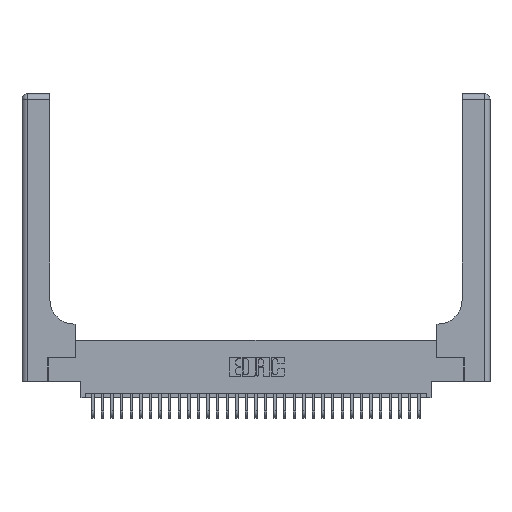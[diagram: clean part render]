
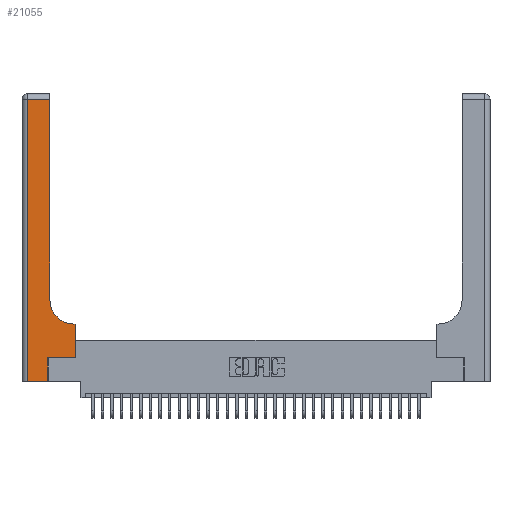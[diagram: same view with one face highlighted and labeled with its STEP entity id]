
A CAD part, top view. The second image highlights one B-rep face of the part: STEP entity #21055.
In plain terms, the highlighted planar face has unit normal (0, 0, 1).
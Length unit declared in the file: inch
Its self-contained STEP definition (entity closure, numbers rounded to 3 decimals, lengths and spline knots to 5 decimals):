
#862 = VECTOR ( 'NONE', #19435, 39.37008 ) ;
#910 = VECTOR ( 'NONE', #25590, 39.37008 ) ;
#3009 = CARTESIAN_POINT ( 'NONE',  ( 0.2915, 3., 0.37 ) ) ;
#3284 = VERTEX_POINT ( 'NONE', #5786 ) ;
#3422 = LINE ( 'NONE', #10126, #9938 ) ;
#4030 = VERTEX_POINT ( 'NONE', #9786 ) ;
#4068 = ORIENTED_EDGE ( 'NONE', *, *, #33892, .T. ) ;
#4175 = CARTESIAN_POINT ( 'NONE',  ( 0.5585, 0.25, 0.37 ) ) ;
#4227 = EDGE_CURVE ( 'NONE', #10998, #13736, #13913, .T. ) ;
#4533 = ORIENTED_EDGE ( 'NONE', *, *, #24375, .T. ) ;
#4627 = EDGE_CURVE ( 'NONE', #26095, #4030, #8307, .T. ) ;
#5786 = CARTESIAN_POINT ( 'NONE',  ( 0.269, 0., 0.37 ) ) ;
#6485 = CARTESIAN_POINT ( 'NONE',  ( 0.06, 3., 0.37 ) ) ;
#7587 = CARTESIAN_POINT ( 'NONE',  ( 0.2915, 0.85, 0.37 ) ) ;
#7722 = CARTESIAN_POINT ( 'NONE',  ( 0., 2.94, 0.37 ) ) ;
#8307 = LINE ( 'NONE', #6485, #910 ) ;
#9136 = CARTESIAN_POINT ( 'NONE',  ( 0.5415, 0.85, 0.37 ) ) ;
#9786 = CARTESIAN_POINT ( 'NONE',  ( 0.06, 0., 0.37 ) ) ;
#9938 = VECTOR ( 'NONE', #26439, 39.37008 ) ;
#10126 = CARTESIAN_POINT ( 'NONE',  ( 0., 0., 0.37 ) ) ;
#10458 = LINE ( 'NONE', #11432, #16880 ) ;
#10578 = ORIENTED_EDGE ( 'NONE', *, *, #33501, .T. ) ;
#10711 = EDGE_LOOP ( 'NONE', ( #10578, #4533, #21641, #4068, #14881, #26355, #33991, #20847, #14951 ) ) ;
#10998 = VERTEX_POINT ( 'NONE', #25466 ) ;
#11432 = CARTESIAN_POINT ( 'NONE',  ( 0.5585, 0.25, 0.37 ) ) ;
#11839 = VECTOR ( 'NONE', #13262, 39.37008 ) ;
#11922 = DIRECTION ( 'NONE',  ( 1., 0., 0. ) ) ;
#12884 = VECTOR ( 'NONE', #16539, 39.37008 ) ;
#13262 = DIRECTION ( 'NONE',  ( -1., 0., 0. ) ) ;
#13263 = CARTESIAN_POINT ( 'NONE',  ( 0.2915, 0.6, 0.37 ) ) ;
#13369 = CARTESIAN_POINT ( 'NONE',  ( 0.269, 0.25, 0.37 ) ) ;
#13731 = LINE ( 'NONE', #30069, #12884 ) ;
#13736 = VERTEX_POINT ( 'NONE', #14645 ) ;
#13913 = LINE ( 'NONE', #13263, #33856 ) ;
#14577 = CARTESIAN_POINT ( 'NONE',  ( 0.06, 2.94, 0.37 ) ) ;
#14645 = CARTESIAN_POINT ( 'NONE',  ( 0.5415, 0.6, 0.37 ) ) ;
#14881 = ORIENTED_EDGE ( 'NONE', *, *, #31077, .T. ) ;
#14951 = ORIENTED_EDGE ( 'NONE', *, *, #28717, .T. ) ;
#14992 = VERTEX_POINT ( 'NONE', #4175 ) ;
#15483 = DIRECTION ( 'NONE',  ( 0., 0., -1. ) ) ;
#16539 = DIRECTION ( 'NONE',  ( 0., 1., 0. ) ) ;
#16730 = CARTESIAN_POINT ( 'NONE',  ( 0.2915, 2.94, 0.37 ) ) ;
#16880 = VECTOR ( 'NONE', #33168, 39.37008 ) ;
#17382 = CARTESIAN_POINT ( 'NONE',  ( 0.269, 0.25, 0.37 ) ) ;
#18393 = FACE_OUTER_BOUND ( 'NONE', #10711, .T. ) ;
#19000 = EDGE_CURVE ( 'NONE', #14992, #10998, #10458, .T. ) ;
#19105 = VERTEX_POINT ( 'NONE', #17382 ) ;
#19435 = DIRECTION ( 'NONE',  ( 0., 1., 0. ) ) ;
#20809 = AXIS2_PLACEMENT_3D ( 'NONE', #26275, #15483, #34441 ) ;
#20847 = ORIENTED_EDGE ( 'NONE', *, *, #4227, .T. ) ;
#21055 = ADVANCED_FACE ( 'NONE', ( #18393 ), #31727, .F. ) ;
#21641 = ORIENTED_EDGE ( 'NONE', *, *, #4627, .T. ) ;
#24375 = EDGE_CURVE ( 'NONE', #25968, #26095, #27145, .T. ) ;
#24632 = LINE ( 'NONE', #13369, #30154 ) ;
#25466 = CARTESIAN_POINT ( 'NONE',  ( 0.5585, 0.6, 0.37 ) ) ;
#25590 = DIRECTION ( 'NONE',  ( 0., -1., 0. ) ) ;
#25968 = VERTEX_POINT ( 'NONE', #16730 ) ;
#26095 = VERTEX_POINT ( 'NONE', #14577 ) ;
#26275 = CARTESIAN_POINT ( 'NONE',  ( 0., 3., 0.37 ) ) ;
#26355 = ORIENTED_EDGE ( 'NONE', *, *, #26493, .T. ) ;
#26439 = DIRECTION ( 'NONE',  ( 1., 0., 0. ) ) ;
#26466 = VERTEX_POINT ( 'NONE', #7587 ) ;
#26493 = EDGE_CURVE ( 'NONE', #19105, #14992, #24632, .T. ) ;
#26898 = DIRECTION ( 'NONE',  ( 1., 0., 0. ) ) ;
#27014 = CIRCLE ( 'NONE', #30104, 0.25 ) ;
#27145 = LINE ( 'NONE', #7722, #11839 ) ;
#28191 = DIRECTION ( 'NONE',  ( 0., 0., -1. ) ) ;
#28717 = EDGE_CURVE ( 'NONE', #13736, #26466, #27014, .T. ) ;
#29124 = LINE ( 'NONE', #3009, #862 ) ;
#29530 = DIRECTION ( 'NONE',  ( -1., 0., 0. ) ) ;
#30069 = CARTESIAN_POINT ( 'NONE',  ( 0.269, 0., 0.37 ) ) ;
#30104 = AXIS2_PLACEMENT_3D ( 'NONE', #9136, #28191, #11922 ) ;
#30154 = VECTOR ( 'NONE', #26898, 39.37008 ) ;
#31077 = EDGE_CURVE ( 'NONE', #3284, #19105, #13731, .T. ) ;
#31727 = PLANE ( 'NONE',  #20809 ) ;
#33168 = DIRECTION ( 'NONE',  ( 0., 1., 0. ) ) ;
#33501 = EDGE_CURVE ( 'NONE', #26466, #25968, #29124, .T. ) ;
#33856 = VECTOR ( 'NONE', #29530, 39.37008 ) ;
#33892 = EDGE_CURVE ( 'NONE', #4030, #3284, #3422, .T. ) ;
#33991 = ORIENTED_EDGE ( 'NONE', *, *, #19000, .T. ) ;
#34441 = DIRECTION ( 'NONE',  ( -1., 0., 0. ) ) ;
